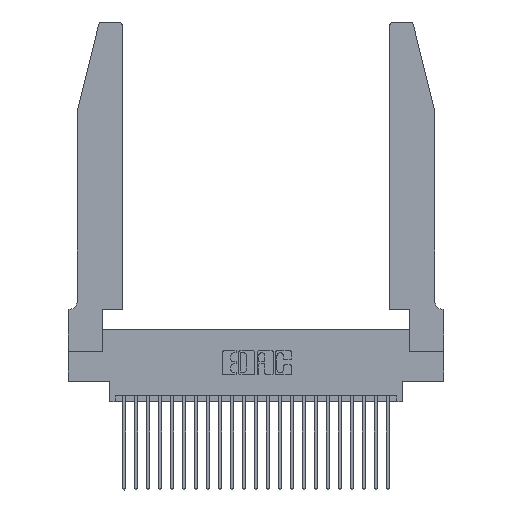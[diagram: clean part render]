
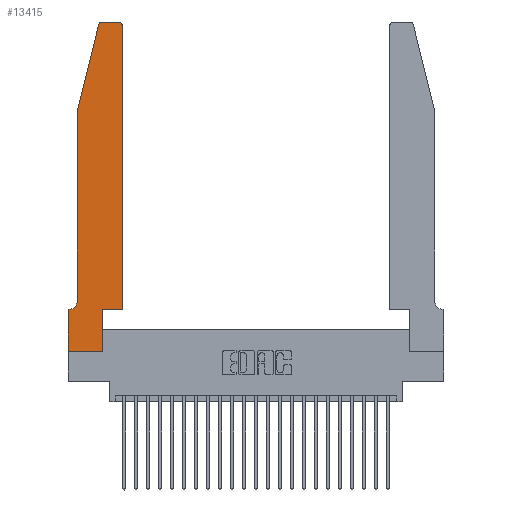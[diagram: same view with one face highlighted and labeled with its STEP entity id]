
A CAD part, top view. The second image highlights one B-rep face of the part: STEP entity #13415.
In plain terms, the highlighted planar face has unit normal (0, 0, 1).
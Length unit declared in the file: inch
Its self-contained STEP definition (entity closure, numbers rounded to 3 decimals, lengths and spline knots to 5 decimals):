
#67 = ORIENTED_EDGE ( 'NONE', *, *, #6643, .T. ) ;
#193 = CARTESIAN_POINT ( 'NONE',  ( 0.2865, 0.35, 0.37 ) ) ;
#384 = CARTESIAN_POINT ( 'NONE',  ( 0.2865, 0., 0.37 ) ) ;
#855 = LINE ( 'NONE', #10739, #8870 ) ;
#1051 = LINE ( 'NONE', #8191, #3222 ) ;
#1325 = CARTESIAN_POINT ( 'NONE',  ( 0., 0.35, 0.37 ) ) ;
#1558 = LINE ( 'NONE', #9488, #11926 ) ;
#1730 = DIRECTION ( 'NONE',  ( 1., 0., 0. ) ) ;
#2456 = CARTESIAN_POINT ( 'NONE',  ( 0.4205, 2.72, 0.37 ) ) ;
#3222 = VECTOR ( 'NONE', #19947, 39.37008 ) ;
#3273 = DIRECTION ( 'NONE',  ( 1., 0., 0. ) ) ;
#3474 = DIRECTION ( 'NONE',  ( 0., 1., 0. ) ) ;
#3938 = AXIS2_PLACEMENT_3D ( 'NONE', #2456, #16938, #9036 ) ;
#3969 = ORIENTED_EDGE ( 'NONE', *, *, #15162, .T. ) ;
#3982 = VERTEX_POINT ( 'NONE', #384 ) ;
#4090 = CARTESIAN_POINT ( 'NONE',  ( 0.4205, 2.75, 0.37 ) ) ;
#4230 = CARTESIAN_POINT ( 'NONE',  ( 0., 0., 0.37 ) ) ;
#4574 = PLANE ( 'NONE',  #11558 ) ;
#4579 = EDGE_CURVE ( 'NONE', #20477, #12866, #1051, .T. ) ;
#4975 = LINE ( 'NONE', #11453, #9590 ) ;
#5201 = VERTEX_POINT ( 'NONE', #13747 ) ;
#5264 = CARTESIAN_POINT ( 'NONE',  ( 0.2865, 0.35, 0.37 ) ) ;
#5294 = LINE ( 'NONE', #5264, #11123 ) ;
#6089 = EDGE_CURVE ( 'NONE', #10721, #5201, #4975, .T. ) ;
#6643 = EDGE_CURVE ( 'NONE', #17590, #3982, #1558, .T. ) ;
#6944 = VECTOR ( 'NONE', #15089, 39.37008 ) ;
#7846 = CARTESIAN_POINT ( 'NONE',  ( 0.0755, 2., 0.37 ) ) ;
#8191 = CARTESIAN_POINT ( 'NONE',  ( 0.4505, 0.35, 0.37 ) ) ;
#8210 = CARTESIAN_POINT ( 'NONE',  ( 0.0055, 0.42, 0.37 ) ) ;
#8292 = DIRECTION ( 'NONE',  ( 0., 0., -1. ) ) ;
#8407 = ORIENTED_EDGE ( 'NONE', *, *, #8827, .T. ) ;
#8827 = EDGE_CURVE ( 'NONE', #16452, #23884, #855, .T. ) ;
#8870 = VECTOR ( 'NONE', #24546, 39.37008 ) ;
#8971 = ORIENTED_EDGE ( 'NONE', *, *, #17661, .T. ) ;
#9021 = CIRCLE ( 'NONE', #20435, 0.07 ) ;
#9036 = DIRECTION ( 'NONE',  ( 1., 0., 0. ) ) ;
#9410 = ORIENTED_EDGE ( 'NONE', *, *, #6089, .T. ) ;
#9488 = CARTESIAN_POINT ( 'NONE',  ( 0., 0., 0.37 ) ) ;
#9590 = VECTOR ( 'NONE', #17252, 39.37008 ) ;
#9635 = DIRECTION ( 'NONE',  ( 0., -1., 0. ) ) ;
#9674 = EDGE_CURVE ( 'NONE', #23884, #10721, #9996, .T. ) ;
#9996 = CIRCLE ( 'NONE', #22614, 0.03 ) ;
#10198 = VECTOR ( 'NONE', #12867, 39.37008 ) ;
#10529 = VECTOR ( 'NONE', #9635, 39.37008 ) ;
#10721 = VERTEX_POINT ( 'NONE', #17318 ) ;
#10733 = ORIENTED_EDGE ( 'NONE', *, *, #21734, .T. ) ;
#10739 = CARTESIAN_POINT ( 'NONE',  ( 0.2605, 2.75, 0.37 ) ) ;
#11123 = VECTOR ( 'NONE', #3474, 39.37008 ) ;
#11258 = VERTEX_POINT ( 'NONE', #22301 ) ;
#11453 = CARTESIAN_POINT ( 'NONE',  ( 0.0755, 2., 0.37 ) ) ;
#11558 = AXIS2_PLACEMENT_3D ( 'NONE', #1325, #24650, #24839 ) ;
#11926 = VECTOR ( 'NONE', #1730, 39.37008 ) ;
#12443 = EDGE_CURVE ( 'NONE', #13997, #17590, #21173, .T. ) ;
#12520 = VERTEX_POINT ( 'NONE', #193 ) ;
#12866 = VERTEX_POINT ( 'NONE', #17155 ) ;
#12867 = DIRECTION ( 'NONE',  ( 1., 0., 0. ) ) ;
#13415 = ADVANCED_FACE ( 'NONE', ( #24825 ), #4574, .T. ) ;
#13747 = CARTESIAN_POINT ( 'NONE',  ( 0.0755, 2., 0.37 ) ) ;
#13997 = VERTEX_POINT ( 'NONE', #14623 ) ;
#14140 = ORIENTED_EDGE ( 'NONE', *, *, #18697, .T. ) ;
#14177 = DIRECTION ( 'NONE',  ( -1., 0., 0. ) ) ;
#14623 = CARTESIAN_POINT ( 'NONE',  ( 0., 0.35, 0.37 ) ) ;
#15089 = DIRECTION ( 'NONE',  ( -1., 0., 0. ) ) ;
#15162 = EDGE_CURVE ( 'NONE', #12520, #20477, #15756, .T. ) ;
#15330 = EDGE_CURVE ( 'NONE', #3982, #12520, #5294, .T. ) ;
#15336 = EDGE_LOOP ( 'NONE', ( #8407, #20923, #9410, #8971, #15584, #10733, #24233, #67, #23361, #3969, #20991, #14140 ) ) ;
#15584 = ORIENTED_EDGE ( 'NONE', *, *, #16964, .T. ) ;
#15756 = LINE ( 'NONE', #16705, #10198 ) ;
#16452 = VERTEX_POINT ( 'NONE', #4090 ) ;
#16705 = CARTESIAN_POINT ( 'NONE',  ( 0.4505, 0.35, 0.37 ) ) ;
#16893 = VERTEX_POINT ( 'NONE', #23082 ) ;
#16938 = DIRECTION ( 'NONE',  ( 0., 0., 1. ) ) ;
#16964 = EDGE_CURVE ( 'NONE', #16893, #11258, #9021, .T. ) ;
#17155 = CARTESIAN_POINT ( 'NONE',  ( 0.4505, 2.72, 0.37 ) ) ;
#17252 = DIRECTION ( 'NONE',  ( -0.239, -0.971, 0. ) ) ;
#17318 = CARTESIAN_POINT ( 'NONE',  ( 0.25487, 2.72718, 0.37 ) ) ;
#17590 = VERTEX_POINT ( 'NONE', #21946 ) ;
#17661 = EDGE_CURVE ( 'NONE', #5201, #16893, #20373, .T. ) ;
#18697 = EDGE_CURVE ( 'NONE', #12866, #16452, #24027, .T. ) ;
#19947 = DIRECTION ( 'NONE',  ( 0., 1., 0. ) ) ;
#20373 = LINE ( 'NONE', #7846, #10529 ) ;
#20435 = AXIS2_PLACEMENT_3D ( 'NONE', #8210, #8292, #14177 ) ;
#20477 = VERTEX_POINT ( 'NONE', #22146 ) ;
#20748 = CARTESIAN_POINT ( 'NONE',  ( 0.284, 2.72, 0.37 ) ) ;
#20923 = ORIENTED_EDGE ( 'NONE', *, *, #9674, .T. ) ;
#20991 = ORIENTED_EDGE ( 'NONE', *, *, #4579, .T. ) ;
#20995 = DIRECTION ( 'NONE',  ( 0., 0., 1. ) ) ;
#21131 = CARTESIAN_POINT ( 'NONE',  ( 0.0755, 0.35, 0.37 ) ) ;
#21173 = LINE ( 'NONE', #4230, #23625 ) ;
#21406 = CARTESIAN_POINT ( 'NONE',  ( 0.284, 2.75, 0.37 ) ) ;
#21683 = LINE ( 'NONE', #21131, #6944 ) ;
#21734 = EDGE_CURVE ( 'NONE', #11258, #13997, #21683, .T. ) ;
#21789 = DIRECTION ( 'NONE',  ( 0., -1., 0. ) ) ;
#21946 = CARTESIAN_POINT ( 'NONE',  ( 0., 0., 0.37 ) ) ;
#22146 = CARTESIAN_POINT ( 'NONE',  ( 0.4505, 0.35, 0.37 ) ) ;
#22301 = CARTESIAN_POINT ( 'NONE',  ( 0.0055, 0.35, 0.37 ) ) ;
#22614 = AXIS2_PLACEMENT_3D ( 'NONE', #20748, #20995, #3273 ) ;
#23082 = CARTESIAN_POINT ( 'NONE',  ( 0.0755, 0.42, 0.37 ) ) ;
#23361 = ORIENTED_EDGE ( 'NONE', *, *, #15330, .T. ) ;
#23625 = VECTOR ( 'NONE', #21789, 39.37008 ) ;
#23884 = VERTEX_POINT ( 'NONE', #21406 ) ;
#24027 = CIRCLE ( 'NONE', #3938, 0.03 ) ;
#24233 = ORIENTED_EDGE ( 'NONE', *, *, #12443, .T. ) ;
#24546 = DIRECTION ( 'NONE',  ( -1., 0., 0. ) ) ;
#24650 = DIRECTION ( 'NONE',  ( 0., 0., 1. ) ) ;
#24825 = FACE_OUTER_BOUND ( 'NONE', #15336, .T. ) ;
#24839 = DIRECTION ( 'NONE',  ( 1., 0., 0. ) ) ;
